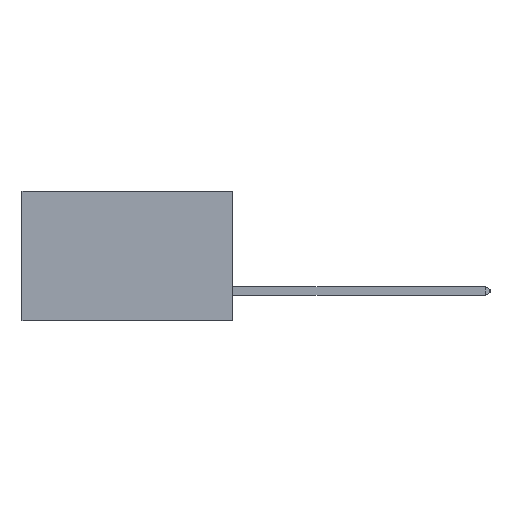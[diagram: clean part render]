
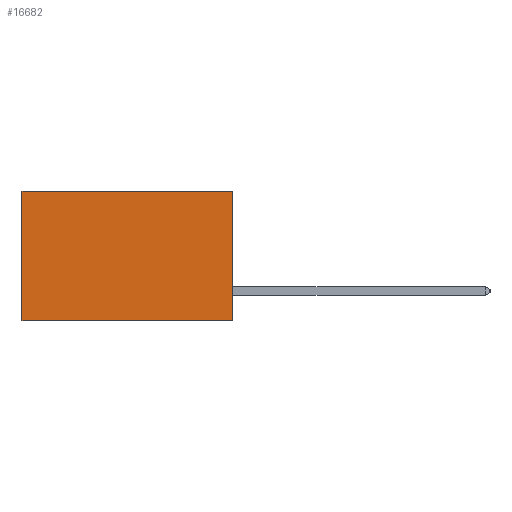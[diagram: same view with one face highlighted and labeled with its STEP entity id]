
A CAD part, left-side view. The second image highlights one B-rep face of the part: STEP entity #16682.
In plain terms, the highlighted planar face has unit normal (-1, 0, 0).
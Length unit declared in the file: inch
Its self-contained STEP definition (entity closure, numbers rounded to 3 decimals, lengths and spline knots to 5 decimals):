
#244 = DIRECTION ( 'NONE',  ( 0., 0., -1. ) ) ;
#639 = CARTESIAN_POINT ( 'NONE',  ( 0.2875, 0., -0.37 ) ) ;
#1610 = DIRECTION ( 'NONE',  ( 1., 0., 0. ) ) ;
#3049 = DIRECTION ( 'NONE',  ( 0., 1., 0. ) ) ;
#3888 = FACE_OUTER_BOUND ( 'NONE', #9292, .T. ) ;
#4033 = VERTEX_POINT ( 'NONE', #18690 ) ;
#4842 = CARTESIAN_POINT ( 'NONE',  ( 0.2875, 0.6, -0.37 ) ) ;
#5969 = CARTESIAN_POINT ( 'NONE',  ( 0.2875, 0.6, 0. ) ) ;
#8841 = AXIS2_PLACEMENT_3D ( 'NONE', #20078, #1610, #17851 ) ;
#9292 = EDGE_LOOP ( 'NONE', ( #25058, #26917, #25575, #19071 ) ) ;
#9706 = LINE ( 'NONE', #639, #22010 ) ;
#10438 = EDGE_CURVE ( 'NONE', #11620, #12338, #24984, .T. ) ;
#11022 = DIRECTION ( 'NONE',  ( 0., 1., 0. ) ) ;
#11026 = VECTOR ( 'NONE', #11022, 39.37008 ) ;
#11620 = VERTEX_POINT ( 'NONE', #29865 ) ;
#12338 = VERTEX_POINT ( 'NONE', #4842 ) ;
#14220 = CARTESIAN_POINT ( 'NONE',  ( 0.2875, 0., 0. ) ) ;
#16682 = ADVANCED_FACE ( 'NONE', ( #3888 ), #29398, .F. ) ;
#17851 = DIRECTION ( 'NONE',  ( 0., 0., -1. ) ) ;
#18427 = LINE ( 'NONE', #14220, #30013 ) ;
#18690 = CARTESIAN_POINT ( 'NONE',  ( 0.2875, 0., -0.37 ) ) ;
#18836 = VECTOR ( 'NONE', #24488, 39.37008 ) ;
#18934 = EDGE_CURVE ( 'NONE', #20796, #11620, #29522, .T. ) ;
#19071 = ORIENTED_EDGE ( 'NONE', *, *, #18934, .T. ) ;
#20078 = CARTESIAN_POINT ( 'NONE',  ( 0.2875, 0., 0. ) ) ;
#20459 = CARTESIAN_POINT ( 'NONE',  ( 0.2875, 0., 0. ) ) ;
#20796 = VERTEX_POINT ( 'NONE', #20459 ) ;
#22010 = VECTOR ( 'NONE', #3049, 39.37008 ) ;
#22318 = EDGE_CURVE ( 'NONE', #20796, #4033, #18427, .T. ) ;
#24488 = DIRECTION ( 'NONE',  ( 0., 0., -1. ) ) ;
#24895 = CARTESIAN_POINT ( 'NONE',  ( 0.2875, 0., 0. ) ) ;
#24984 = LINE ( 'NONE', #5969, #18836 ) ;
#25058 = ORIENTED_EDGE ( 'NONE', *, *, #10438, .T. ) ;
#25575 = ORIENTED_EDGE ( 'NONE', *, *, #22318, .F. ) ;
#26917 = ORIENTED_EDGE ( 'NONE', *, *, #27528, .F. ) ;
#27528 = EDGE_CURVE ( 'NONE', #4033, #12338, #9706, .T. ) ;
#29398 = PLANE ( 'NONE',  #8841 ) ;
#29522 = LINE ( 'NONE', #24895, #11026 ) ;
#29865 = CARTESIAN_POINT ( 'NONE',  ( 0.2875, 0.6, 0. ) ) ;
#30013 = VECTOR ( 'NONE', #244, 39.37008 ) ;
